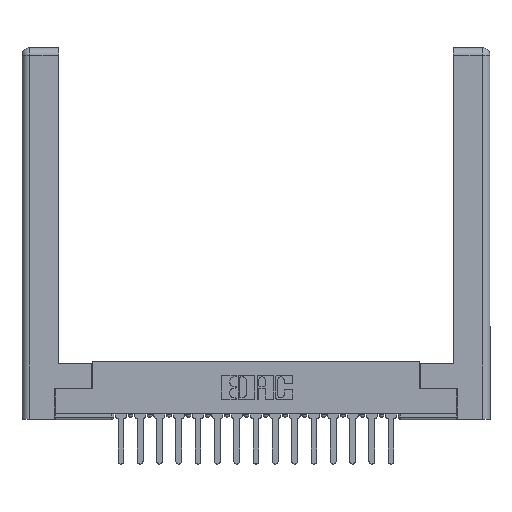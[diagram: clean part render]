
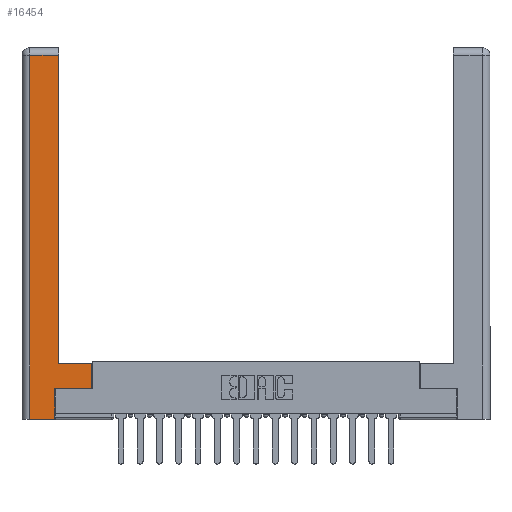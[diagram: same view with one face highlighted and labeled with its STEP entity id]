
A CAD part, top view. The second image highlights one B-rep face of the part: STEP entity #16454.
In plain terms, the highlighted planar face has unit normal (0, 0, 1).
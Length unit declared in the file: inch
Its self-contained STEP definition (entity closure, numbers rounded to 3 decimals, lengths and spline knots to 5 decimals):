
#1172 = DIRECTION ( 'NONE',  ( 1., 0., 0. ) ) ;
#1277 = EDGE_LOOP ( 'NONE', ( #8854, #15940, #16388, #18433, #4637, #13189, #13700, #12702 ) ) ;
#1671 = DIRECTION ( 'NONE',  ( 0., 1., 0. ) ) ;
#2865 = VERTEX_POINT ( 'NONE', #10169 ) ;
#2885 = DIRECTION ( 'NONE',  ( 0., 1., 0. ) ) ;
#3105 = CARTESIAN_POINT ( 'NONE',  ( 0.295, 3., 0. ) ) ;
#3186 = CARTESIAN_POINT ( 'NONE',  ( 0.265, 0.245, 0. ) ) ;
#3503 = EDGE_CURVE ( 'NONE', #14230, #15133, #6955, .T. ) ;
#3596 = LINE ( 'NONE', #18195, #12397 ) ;
#3752 = CARTESIAN_POINT ( 'NONE',  ( 0.0615, 2.94, 0. ) ) ;
#3977 = PLANE ( 'NONE',  #7093 ) ;
#4128 = EDGE_CURVE ( 'NONE', #5716, #6184, #15970, .T. ) ;
#4637 = ORIENTED_EDGE ( 'NONE', *, *, #9265, .T. ) ;
#4669 = VERTEX_POINT ( 'NONE', #14704 ) ;
#5236 = DIRECTION ( 'NONE',  ( 1., 0., 0. ) ) ;
#5432 = CARTESIAN_POINT ( 'NONE',  ( 0.565, 0.245, 0. ) ) ;
#5529 = CARTESIAN_POINT ( 'NONE',  ( 0.0615, 2.94, 0. ) ) ;
#5565 = VECTOR ( 'NONE', #2885, 39.37008 ) ;
#5716 = VERTEX_POINT ( 'NONE', #5529 ) ;
#6052 = DIRECTION ( 'NONE',  ( 0., -1., 0. ) ) ;
#6184 = VERTEX_POINT ( 'NONE', #19063 ) ;
#6955 = LINE ( 'NONE', #9116, #11113 ) ;
#7093 = AXIS2_PLACEMENT_3D ( 'NONE', #15954, #19046, #18908 ) ;
#7157 = VECTOR ( 'NONE', #6052, 39.37008 ) ;
#7601 = CARTESIAN_POINT ( 'NONE',  ( 0.0615, 0., 0. ) ) ;
#7666 = CARTESIAN_POINT ( 'NONE',  ( 0.295, 2.94, 0. ) ) ;
#7883 = VECTOR ( 'NONE', #14242, 39.37008 ) ;
#8529 = EDGE_CURVE ( 'NONE', #6184, #4669, #18633, .T. ) ;
#8601 = LINE ( 'NONE', #3105, #17184 ) ;
#8854 = ORIENTED_EDGE ( 'NONE', *, *, #14973, .T. ) ;
#9116 = CARTESIAN_POINT ( 'NONE',  ( 0.295, 0.45, 0. ) ) ;
#9265 = EDGE_CURVE ( 'NONE', #4669, #14294, #13416, .T. ) ;
#9319 = VECTOR ( 'NONE', #1172, 39.37008 ) ;
#9884 = EDGE_CURVE ( 'NONE', #16715, #5716, #10879, .T. ) ;
#10169 = CARTESIAN_POINT ( 'NONE',  ( 0.565, 0.245, 0. ) ) ;
#10795 = CARTESIAN_POINT ( 'NONE',  ( 0.295, 0.45, 0. ) ) ;
#10879 = LINE ( 'NONE', #3752, #7883 ) ;
#11113 = VECTOR ( 'NONE', #14941, 39.37008 ) ;
#11238 = VECTOR ( 'NONE', #5236, 39.37008 ) ;
#11405 = LINE ( 'NONE', #5432, #11238 ) ;
#11471 = CARTESIAN_POINT ( 'NONE',  ( 0.265, 0., 0. ) ) ;
#11770 = FACE_OUTER_BOUND ( 'NONE', #1277, .T. ) ;
#11923 = CARTESIAN_POINT ( 'NONE',  ( 0.565, 0.45, 0. ) ) ;
#12397 = VECTOR ( 'NONE', #13634, 39.37008 ) ;
#12702 = ORIENTED_EDGE ( 'NONE', *, *, #3503, .T. ) ;
#13189 = ORIENTED_EDGE ( 'NONE', *, *, #15236, .T. ) ;
#13416 = LINE ( 'NONE', #17670, #5565 ) ;
#13634 = DIRECTION ( 'NONE',  ( 0., 1., 0. ) ) ;
#13700 = ORIENTED_EDGE ( 'NONE', *, *, #17958, .T. ) ;
#14230 = VERTEX_POINT ( 'NONE', #11923 ) ;
#14242 = DIRECTION ( 'NONE',  ( -1., 0., 0. ) ) ;
#14294 = VERTEX_POINT ( 'NONE', #3186 ) ;
#14704 = CARTESIAN_POINT ( 'NONE',  ( 0.265, 0., 0. ) ) ;
#14941 = DIRECTION ( 'NONE',  ( -1., 0., 0. ) ) ;
#14973 = EDGE_CURVE ( 'NONE', #15133, #16715, #8601, .T. ) ;
#15133 = VERTEX_POINT ( 'NONE', #10795 ) ;
#15236 = EDGE_CURVE ( 'NONE', #14294, #2865, #11405, .T. ) ;
#15940 = ORIENTED_EDGE ( 'NONE', *, *, #9884, .T. ) ;
#15954 = CARTESIAN_POINT ( 'NONE',  ( 0., 0., 0. ) ) ;
#15970 = LINE ( 'NONE', #7601, #7157 ) ;
#16388 = ORIENTED_EDGE ( 'NONE', *, *, #4128, .T. ) ;
#16454 = ADVANCED_FACE ( 'NONE', ( #11770 ), #3977, .F. ) ;
#16715 = VERTEX_POINT ( 'NONE', #7666 ) ;
#17184 = VECTOR ( 'NONE', #1671, 39.37008 ) ;
#17670 = CARTESIAN_POINT ( 'NONE',  ( 0.265, 0.245, 0. ) ) ;
#17958 = EDGE_CURVE ( 'NONE', #2865, #14230, #3596, .T. ) ;
#18195 = CARTESIAN_POINT ( 'NONE',  ( 0.565, 0.45, 0. ) ) ;
#18433 = ORIENTED_EDGE ( 'NONE', *, *, #8529, .T. ) ;
#18633 = LINE ( 'NONE', #11471, #9319 ) ;
#18908 = DIRECTION ( 'NONE',  ( -1., 0., 0. ) ) ;
#19046 = DIRECTION ( 'NONE',  ( 0., 0., -1. ) ) ;
#19063 = CARTESIAN_POINT ( 'NONE',  ( 0.0615, 0., 0. ) ) ;
